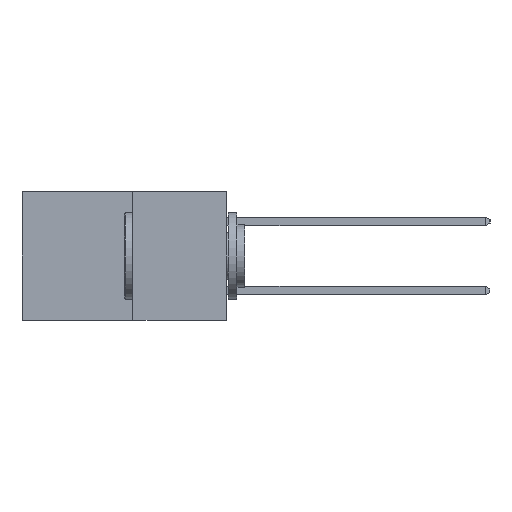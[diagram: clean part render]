
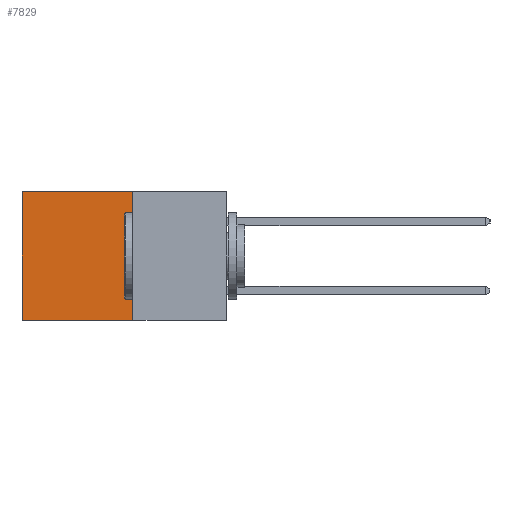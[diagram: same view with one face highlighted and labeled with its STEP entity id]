
A CAD part, left-side view. The second image highlights one B-rep face of the part: STEP entity #7829.
In plain terms, the highlighted planar face has unit normal (-1, 0, 0).
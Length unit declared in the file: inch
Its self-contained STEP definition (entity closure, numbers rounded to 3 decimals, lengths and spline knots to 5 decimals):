
#175 = ORIENTED_EDGE ( 'NONE', *, *, #2784, .F. ) ;
#206 = EDGE_CURVE ( 'NONE', #383, #2806, #7563, .T. ) ;
#238 = EDGE_LOOP ( 'NONE', ( #1944, #175, #2172, #2407 ) ) ;
#383 = VERTEX_POINT ( 'NONE', #1204 ) ;
#1204 = CARTESIAN_POINT ( 'NONE',  ( 0.277, 0.27, 0. ) ) ;
#1557 = LINE ( 'NONE', #4593, #3482 ) ;
#1601 = EDGE_CURVE ( 'NONE', #383, #5700, #1557, .T. ) ;
#1944 = ORIENTED_EDGE ( 'NONE', *, *, #6854, .T. ) ;
#2046 = CARTESIAN_POINT ( 'NONE',  ( 0.277, 0.59, -0.37 ) ) ;
#2048 = DIRECTION ( 'NONE',  ( 0., 1., 0. ) ) ;
#2172 = ORIENTED_EDGE ( 'NONE', *, *, #1601, .F. ) ;
#2198 = CARTESIAN_POINT ( 'NONE',  ( 0.277, 0.59, -0.37 ) ) ;
#2407 = ORIENTED_EDGE ( 'NONE', *, *, #206, .T. ) ;
#2784 = EDGE_CURVE ( 'NONE', #5700, #5212, #9813, .T. ) ;
#2806 = VERTEX_POINT ( 'NONE', #8426 ) ;
#3390 = VECTOR ( 'NONE', #7714, 39.37008 ) ;
#3482 = VECTOR ( 'NONE', #6805, 39.37008 ) ;
#3605 = DIRECTION ( 'NONE',  ( 1., 0., 0. ) ) ;
#4593 = CARTESIAN_POINT ( 'NONE',  ( 0.277, 0.27, -0.37 ) ) ;
#5040 = VECTOR ( 'NONE', #9328, 39.37008 ) ;
#5212 = VERTEX_POINT ( 'NONE', #2046 ) ;
#5700 = VERTEX_POINT ( 'NONE', #8085 ) ;
#6012 = CARTESIAN_POINT ( 'NONE',  ( 0.277, 0.27, -0.37 ) ) ;
#6805 = DIRECTION ( 'NONE',  ( 0., 0., -1. ) ) ;
#6854 = EDGE_CURVE ( 'NONE', #2806, #5212, #7115, .T. ) ;
#7115 = LINE ( 'NONE', #2198, #5040 ) ;
#7552 = PLANE ( 'NONE',  #8933 ) ;
#7563 = LINE ( 'NONE', #9333, #3390 ) ;
#7714 = DIRECTION ( 'NONE',  ( 0., 1., 0. ) ) ;
#7822 = VECTOR ( 'NONE', #2048, 39.37008 ) ;
#7829 = ADVANCED_FACE ( 'NONE', ( #9634 ), #7552, .F. ) ;
#8085 = CARTESIAN_POINT ( 'NONE',  ( 0.277, 0.27, -0.37 ) ) ;
#8358 = CARTESIAN_POINT ( 'NONE',  ( 0.277, 0.27, -0.37 ) ) ;
#8426 = CARTESIAN_POINT ( 'NONE',  ( 0.277, 0.59, 0. ) ) ;
#8933 = AXIS2_PLACEMENT_3D ( 'NONE', #8358, #3605, #9139 ) ;
#9139 = DIRECTION ( 'NONE',  ( 0., 0., -1. ) ) ;
#9328 = DIRECTION ( 'NONE',  ( 0., 0., -1. ) ) ;
#9333 = CARTESIAN_POINT ( 'NONE',  ( 0.277, 0.27, 0. ) ) ;
#9634 = FACE_OUTER_BOUND ( 'NONE', #238, .T. ) ;
#9813 = LINE ( 'NONE', #6012, #7822 ) ;
